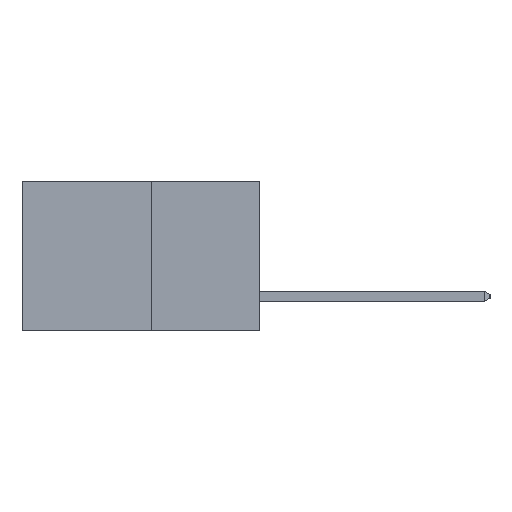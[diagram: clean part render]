
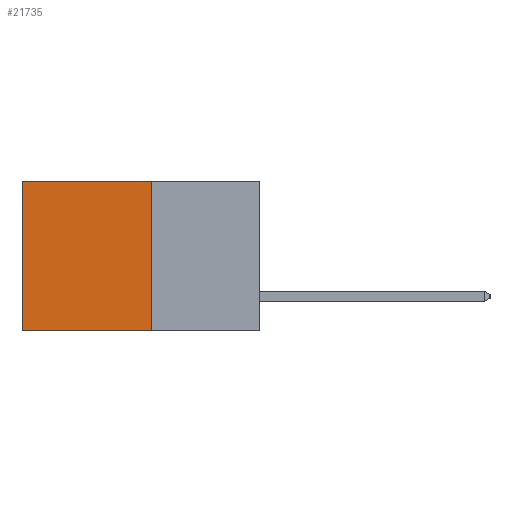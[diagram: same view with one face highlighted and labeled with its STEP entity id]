
A CAD part, left-side view. The second image highlights one B-rep face of the part: STEP entity #21735.
In plain terms, the highlighted planar face has unit normal (-1, 0, 0).
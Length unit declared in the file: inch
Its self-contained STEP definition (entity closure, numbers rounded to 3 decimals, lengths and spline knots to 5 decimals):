
#687 = DIRECTION ( 'NONE',  ( 0., 1., 0. ) ) ;
#1061 = VERTEX_POINT ( 'NONE', #7577 ) ;
#1842 = LINE ( 'NONE', #4048, #14922 ) ;
#2216 = CARTESIAN_POINT ( 'NONE',  ( 0.277, 0.27, -0.37 ) ) ;
#2415 = PLANE ( 'NONE',  #2560 ) ;
#2560 = AXIS2_PLACEMENT_3D ( 'NONE', #4132, #5893, #17746 ) ;
#2668 = VERTEX_POINT ( 'NONE', #2819 ) ;
#2819 = CARTESIAN_POINT ( 'NONE',  ( 0.277, 0.59, 0. ) ) ;
#3180 = EDGE_CURVE ( 'NONE', #2668, #9450, #13152, .T. ) ;
#4047 = CARTESIAN_POINT ( 'NONE',  ( 0.277, 0.59, -0.37 ) ) ;
#4048 = CARTESIAN_POINT ( 'NONE',  ( 0.277, 0.27, 0. ) ) ;
#4132 = CARTESIAN_POINT ( 'NONE',  ( 0.277, 0.27, -0.37 ) ) ;
#5724 = DIRECTION ( 'NONE',  ( 0., 0., -1. ) ) ;
#5858 = EDGE_CURVE ( 'NONE', #12909, #9450, #6688, .T. ) ;
#5893 = DIRECTION ( 'NONE',  ( 1., 0., 0. ) ) ;
#6688 = LINE ( 'NONE', #13260, #19585 ) ;
#7577 = CARTESIAN_POINT ( 'NONE',  ( 0.277, 0.27, 0. ) ) ;
#7881 = ORIENTED_EDGE ( 'NONE', *, *, #3180, .T. ) ;
#9180 = EDGE_CURVE ( 'NONE', #1061, #12909, #14551, .T. ) ;
#9450 = VERTEX_POINT ( 'NONE', #4047 ) ;
#10010 = VECTOR ( 'NONE', #5724, 39.37008 ) ;
#11892 = ORIENTED_EDGE ( 'NONE', *, *, #9180, .F. ) ;
#12909 = VERTEX_POINT ( 'NONE', #16081 ) ;
#13121 = DIRECTION ( 'NONE',  ( 0., 1., 0. ) ) ;
#13152 = LINE ( 'NONE', #20234, #21427 ) ;
#13260 = CARTESIAN_POINT ( 'NONE',  ( 0.277, 0.27, -0.37 ) ) ;
#14551 = LINE ( 'NONE', #2216, #10010 ) ;
#14855 = ORIENTED_EDGE ( 'NONE', *, *, #21716, .T. ) ;
#14922 = VECTOR ( 'NONE', #687, 39.37008 ) ;
#16081 = CARTESIAN_POINT ( 'NONE',  ( 0.277, 0.27, -0.37 ) ) ;
#16597 = ORIENTED_EDGE ( 'NONE', *, *, #5858, .F. ) ;
#17746 = DIRECTION ( 'NONE',  ( 0., 0., -1. ) ) ;
#19585 = VECTOR ( 'NONE', #13121, 39.37008 ) ;
#19831 = FACE_OUTER_BOUND ( 'NONE', #21212, .T. ) ;
#20234 = CARTESIAN_POINT ( 'NONE',  ( 0.277, 0.59, -0.37 ) ) ;
#20720 = DIRECTION ( 'NONE',  ( 0., 0., -1. ) ) ;
#21212 = EDGE_LOOP ( 'NONE', ( #7881, #16597, #11892, #14855 ) ) ;
#21427 = VECTOR ( 'NONE', #20720, 39.37008 ) ;
#21716 = EDGE_CURVE ( 'NONE', #1061, #2668, #1842, .T. ) ;
#21735 = ADVANCED_FACE ( 'NONE', ( #19831 ), #2415, .F. ) ;
